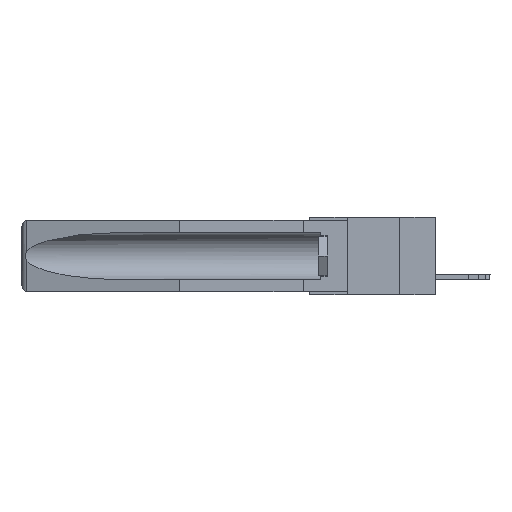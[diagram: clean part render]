
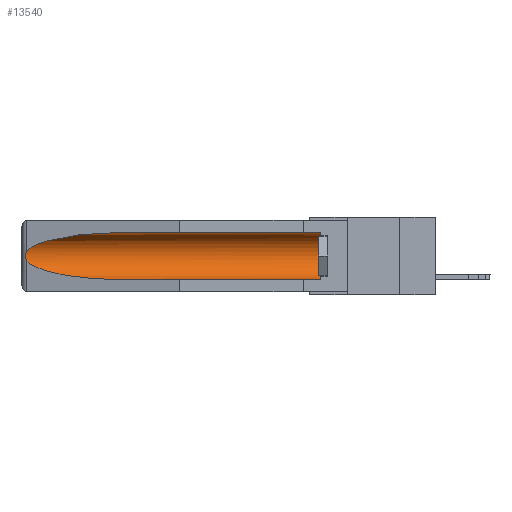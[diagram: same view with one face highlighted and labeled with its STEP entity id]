
A CAD part, left-side view. The second image highlights one B-rep face of the part: STEP entity #13540.
In plain terms, the highlighted cylindrical face has radius 2.857 mm (diameter 5.715 mm), a partial arc.
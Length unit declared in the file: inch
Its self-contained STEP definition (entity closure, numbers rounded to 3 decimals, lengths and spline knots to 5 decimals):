
#395 = ORIENTED_EDGE ( 'NONE', *, *, #8390, .F. ) ;
#452 = CARTESIAN_POINT ( 'NONE',  ( 0.155, 0.126, -0.284 ) ) ;
#747 = CARTESIAN_POINT ( 'NONE',  ( 0.155, 1.07973, -0.059 ) ) ;
#1921 = EDGE_LOOP ( 'NONE', ( #13263, #17953, #22069, #395, #18898, #4796 ) ) ;
#2833 = CARTESIAN_POINT ( 'NONE',  ( 0.155, 0.126, -0.1715 ) ) ;
#3824 = EDGE_CURVE ( 'NONE', #19512, #19394, #21894, .T. ) ;
#4085 = CARTESIAN_POINT ( 'NONE',  ( 0.2673, 1.5327, -0.16383 ) ) ;
#4511 = CARTESIAN_POINT ( 'NONE',  ( 0.155, 0.126, -0.059 ) ) ;
#4796 = ORIENTED_EDGE ( 'NONE', *, *, #20576, .T. ) ;
#5345 = CARTESIAN_POINT ( 'NONE',  ( 0.155, 1.07973, -0.284 ) ) ;
#6072 = DIRECTION ( 'NONE',  ( 0., 0., 1. ) ) ;
#6501 = CARTESIAN_POINT ( 'NONE',  ( 0.26537, 1.52718, -0.19328 ) ) ;
#7893 = B_SPLINE_CURVE_WITH_KNOTS ( 'NONE', 3,
 ( #16394, #8359, #20722, #4085, #11761, #18446, #25075, #24735, #8271, #12308 ),
 .UNSPECIFIED., .F., .F.,
 ( 4, 2, 2, 2, 4 ),
 ( 0., 0.00029, 0.00058, 0.00087, 0.00117 ),
 .UNSPECIFIED. ) ;
#8195 = FACE_OUTER_BOUND ( 'NONE', #1921, .T. ) ;
#8240 = CARTESIAN_POINT ( 'NONE',  ( 0.155, -0.30754, -0.284 ) ) ;
#8271 = CARTESIAN_POINT ( 'NONE',  ( 0.26597, 1.5296, -0.19026 ) ) ;
#8359 = CARTESIAN_POINT ( 'NONE',  ( 0.26597, 1.52961, -0.15275 ) ) ;
#8390 = EDGE_CURVE ( 'NONE', #13450, #19394, #19064, .T. ) ;
#10376 = DIRECTION ( 'NONE',  ( 0., 1., 0. ) ) ;
#11115 = DIRECTION ( 'NONE',  ( 0., 0., 1. ) ) ;
#11330 = CARTESIAN_POINT ( 'NONE',  ( 0.25451, 1.48313, -0.09465 ) ) ;
#11761 = CARTESIAN_POINT ( 'NONE',  ( 0.2675, 1.53308, -0.16763 ) ) ;
#11996 = CIRCLE ( 'NONE', #23081, 0.1125 ) ;
#12308 = CARTESIAN_POINT ( 'NONE',  ( 0.26537, 1.52718, -0.19328 ) ) ;
#12854 = CYLINDRICAL_SURFACE ( 'NONE', #21403, 0.1125 ) ;
#13263 = ORIENTED_EDGE ( 'NONE', *, *, #13991, .T. ) ;
#13450 = VERTEX_POINT ( 'NONE', #452 ) ;
#13540 = ADVANCED_FACE ( 'NONE', ( #8195 ), #12854, .F. ) ;
#13991 = EDGE_CURVE ( 'NONE', #15927, #16635, #22729, .T. ) ;
#14606 = VERTEX_POINT ( 'NONE', #4511 ) ;
#15508 = DIRECTION ( 'NONE',  ( 0., 1., 0. ) ) ;
#15927 = VERTEX_POINT ( 'NONE', #24523 ) ;
#16005 = EDGE_CURVE ( 'NONE', #16635, #19512, #7893, .T. ) ;
#16394 = CARTESIAN_POINT ( 'NONE',  ( 0.26537, 1.52718, -0.14972 ) ) ;
#16635 = VERTEX_POINT ( 'NONE', #20528 ) ;
#17953 = ORIENTED_EDGE ( 'NONE', *, *, #16005, .T. ) ;
#18446 = CARTESIAN_POINT ( 'NONE',  ( 0.2675, 1.53308, -0.17534 ) ) ;
#18898 = ORIENTED_EDGE ( 'NONE', *, *, #20519, .T. ) ;
#19064 = LINE ( 'NONE', #8240, #21309 ) ;
#19109 = CARTESIAN_POINT ( 'NONE',  ( 0.155, 1.07973, -0.284 ) ) ;
#19394 = VERTEX_POINT ( 'NONE', #19109 ) ;
#19496 = CARTESIAN_POINT ( 'NONE',  ( 0.26537, 1.52718, -0.14972 ) ) ;
#19512 = VERTEX_POINT ( 'NONE', #6501 ) ;
#20519 = EDGE_CURVE ( 'NONE', #13450, #14606, #11996, .T. ) ;
#20528 = CARTESIAN_POINT ( 'NONE',  ( 0.26537, 1.52718, -0.14972 ) ) ;
#20576 = EDGE_CURVE ( 'NONE', #14606, #15927, #26944, .T. ) ;
#20722 = CARTESIAN_POINT ( 'NONE',  ( 0.26654, 1.53092, -0.15636 ) ) ;
#21309 = VECTOR ( 'NONE', #21972, 39.37008 ) ;
#21403 = AXIS2_PLACEMENT_3D ( 'NONE', #26748, #10376, #6072 ) ;
#21710 = CARTESIAN_POINT ( 'NONE',  ( 0.21114, 1.30732, -0.284 ) ) ;
#21894 =( BOUNDED_CURVE ( )  B_SPLINE_CURVE ( 3, ( #26082, #23717, #21710, #5345 ),
 .UNSPECIFIED., .F., .F. ) 
 B_SPLINE_CURVE_WITH_KNOTS ( ( 4, 4 ),
 ( 0.1948, 1.5708 ),
 .UNSPECIFIED. ) 
 CURVE ( )  GEOMETRIC_REPRESENTATION_ITEM ( )  RATIONAL_B_SPLINE_CURVE ( ( 1., 0.848, 0.848, 1. ) ) 
 REPRESENTATION_ITEM ( '' )  );
#21972 = DIRECTION ( 'NONE',  ( 0., 1., 0. ) ) ;
#22069 = ORIENTED_EDGE ( 'NONE', *, *, #3824, .T. ) ;
#22729 =( BOUNDED_CURVE ( )  B_SPLINE_CURVE ( 3, ( #747, #23938, #11330, #19496 ),
 .UNSPECIFIED., .F., .F. ) 
 B_SPLINE_CURVE_WITH_KNOTS ( ( 4, 4 ),
 ( 4.71239, 6.08839 ),
 .UNSPECIFIED. ) 
 CURVE ( )  GEOMETRIC_REPRESENTATION_ITEM ( )  RATIONAL_B_SPLINE_CURVE ( ( 1., 0.848, 0.848, 1. ) ) 
 REPRESENTATION_ITEM ( '' )  );
#23081 = AXIS2_PLACEMENT_3D ( 'NONE', #2833, #23721, #11115 ) ;
#23432 = CARTESIAN_POINT ( 'NONE',  ( 0.155, -0.30754, -0.059 ) ) ;
#23680 = VECTOR ( 'NONE', #15508, 39.37008 ) ;
#23717 = CARTESIAN_POINT ( 'NONE',  ( 0.25451, 1.48313, -0.24835 ) ) ;
#23721 = DIRECTION ( 'NONE',  ( 0., -1., 0. ) ) ;
#23938 = CARTESIAN_POINT ( 'NONE',  ( 0.21114, 1.30732, -0.059 ) ) ;
#24523 = CARTESIAN_POINT ( 'NONE',  ( 0.155, 1.07973, -0.059 ) ) ;
#24735 = CARTESIAN_POINT ( 'NONE',  ( 0.26655, 1.53094, -0.18657 ) ) ;
#25075 = CARTESIAN_POINT ( 'NONE',  ( 0.2673, 1.53269, -0.17917 ) ) ;
#26082 = CARTESIAN_POINT ( 'NONE',  ( 0.26537, 1.52718, -0.19328 ) ) ;
#26748 = CARTESIAN_POINT ( 'NONE',  ( 0.155, -0.30754, -0.1715 ) ) ;
#26944 = LINE ( 'NONE', #23432, #23680 ) ;
